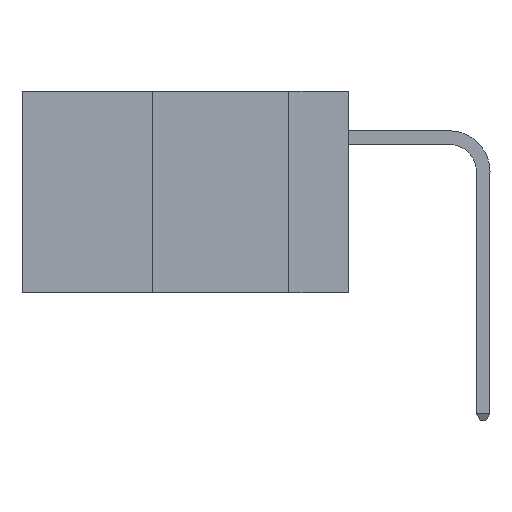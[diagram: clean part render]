
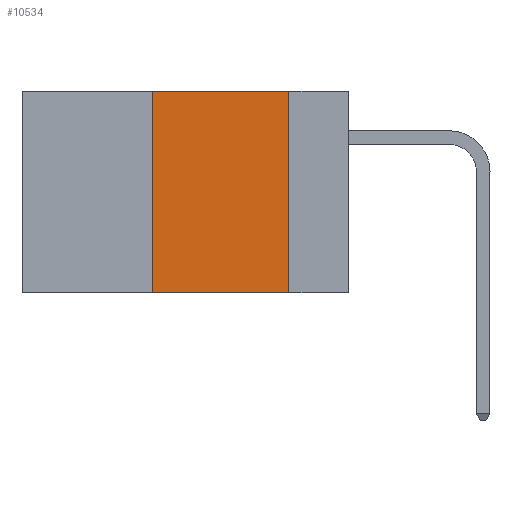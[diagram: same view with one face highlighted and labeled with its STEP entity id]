
A CAD part, left-side view. The second image highlights one B-rep face of the part: STEP entity #10534.
In plain terms, the highlighted planar face has unit normal (-1, 0, 0).
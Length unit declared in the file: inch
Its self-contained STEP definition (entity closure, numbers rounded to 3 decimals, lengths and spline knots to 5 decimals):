
#480 = CARTESIAN_POINT ( 'NONE',  ( 0., 0.11, 0. ) ) ;
#679 = DIRECTION ( 'NONE',  ( 0., 0., -1. ) ) ;
#1357 = DIRECTION ( 'NONE',  ( 0., 0., 1. ) ) ;
#1808 = LINE ( 'NONE', #13125, #12155 ) ;
#2209 = LINE ( 'NONE', #11371, #15274 ) ;
#3025 = CARTESIAN_POINT ( 'NONE',  ( 0., 0.36, -0.37 ) ) ;
#3200 = PLANE ( 'NONE',  #14526 ) ;
#3237 = FACE_OUTER_BOUND ( 'NONE', #10487, .T. ) ;
#4911 = EDGE_CURVE ( 'NONE', #11552, #15827, #15587, .T. ) ;
#5443 = VECTOR ( 'NONE', #12699, 39.37008 ) ;
#5770 = CARTESIAN_POINT ( 'NONE',  ( 0., 0.6, 0. ) ) ;
#5858 = LINE ( 'NONE', #11301, #5443 ) ;
#6483 = CARTESIAN_POINT ( 'NONE',  ( 0., 0.6, 0. ) ) ;
#7084 = VERTEX_POINT ( 'NONE', #16145 ) ;
#7733 = DIRECTION ( 'NONE',  ( 0., -1., 0. ) ) ;
#8132 = DIRECTION ( 'NONE',  ( 0., 0., -1. ) ) ;
#8160 = CARTESIAN_POINT ( 'NONE',  ( 0., 0.36, 0. ) ) ;
#8314 = DIRECTION ( 'NONE',  ( 1., 0., 0. ) ) ;
#8335 = VECTOR ( 'NONE', #7733, 39.37008 ) ;
#10487 = EDGE_LOOP ( 'NONE', ( #14870, #13267, #12007, #13196 ) ) ;
#10534 = ADVANCED_FACE ( 'NONE', ( #3237 ), #3200, .F. ) ;
#11059 = EDGE_CURVE ( 'NONE', #15053, #11552, #2209, .T. ) ;
#11301 = CARTESIAN_POINT ( 'NONE',  ( 0., 0.6, -0.37 ) ) ;
#11371 = CARTESIAN_POINT ( 'NONE',  ( 0., 0.36, 0. ) ) ;
#11552 = VERTEX_POINT ( 'NONE', #8160 ) ;
#12007 = ORIENTED_EDGE ( 'NONE', *, *, #11059, .F. ) ;
#12155 = VECTOR ( 'NONE', #8132, 39.37008 ) ;
#12699 = DIRECTION ( 'NONE',  ( 0., -1., 0. ) ) ;
#13125 = CARTESIAN_POINT ( 'NONE',  ( 0., 0.11, 0. ) ) ;
#13196 = ORIENTED_EDGE ( 'NONE', *, *, #14349, .T. ) ;
#13267 = ORIENTED_EDGE ( 'NONE', *, *, #4911, .F. ) ;
#14349 = EDGE_CURVE ( 'NONE', #15053, #7084, #5858, .T. ) ;
#14526 = AXIS2_PLACEMENT_3D ( 'NONE', #5770, #8314, #679 ) ;
#14870 = ORIENTED_EDGE ( 'NONE', *, *, #15057, .F. ) ;
#15053 = VERTEX_POINT ( 'NONE', #3025 ) ;
#15057 = EDGE_CURVE ( 'NONE', #15827, #7084, #1808, .T. ) ;
#15274 = VECTOR ( 'NONE', #1357, 39.37008 ) ;
#15587 = LINE ( 'NONE', #6483, #8335 ) ;
#15827 = VERTEX_POINT ( 'NONE', #480 ) ;
#16145 = CARTESIAN_POINT ( 'NONE',  ( 0., 0.11, -0.37 ) ) ;
